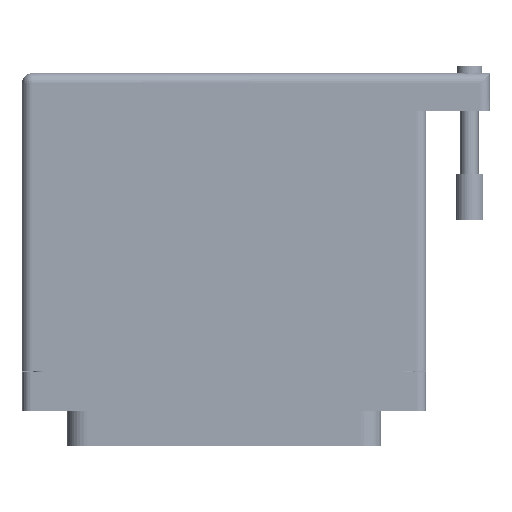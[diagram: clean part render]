
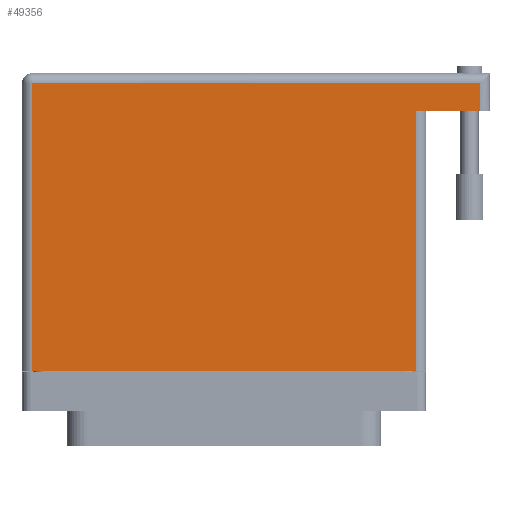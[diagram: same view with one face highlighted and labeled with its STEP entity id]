
A CAD part, front view. The second image highlights one B-rep face of the part: STEP entity #49356.
In plain terms, the highlighted face is planar.
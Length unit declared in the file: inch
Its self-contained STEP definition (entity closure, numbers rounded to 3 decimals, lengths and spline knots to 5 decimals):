
#3631 = CARTESIAN_POINT ( 'NONE',  ( 1.8125, 1.674, 0.765 ) ) ;
#5376 = DIRECTION ( 'NONE',  ( -1., 0., 0. ) ) ;
#6197 = ORIENTED_EDGE ( 'NONE', *, *, #26275, .F. ) ;
#10442 = CARTESIAN_POINT ( 'NONE',  ( -1.3775, -0.1, 0.765 ) ) ;
#16301 = CARTESIAN_POINT ( 'NONE',  ( -1.3775, 1.86, 0.765 ) ) ;
#18499 = CARTESIAN_POINT ( 'NONE',  ( -1.3775, 1.93, 0.765 ) ) ;
#18827 = VERTEX_POINT ( 'NONE', #66549 ) ;
#19673 = FACE_OUTER_BOUND ( 'NONE', #25398, .T. ) ;
#20328 = ORIENTED_EDGE ( 'NONE', *, *, #23964, .T. ) ;
#21923 = VECTOR ( 'NONE', #41911, 39.37008 ) ;
#23964 = EDGE_CURVE ( 'NONE', #54976, #90650, #58745, .T. ) ;
#24410 = VERTEX_POINT ( 'NONE', #43535 ) ;
#25398 = EDGE_LOOP ( 'NONE', ( #61426, #30986, #6197, #43374, #41675, #20328 ) ) ;
#26275 = EDGE_CURVE ( 'NONE', #24410, #18827, #43807, .T. ) ;
#28622 = CARTESIAN_POINT ( 'NONE',  ( -1.3075, 1.86, 0.765 ) ) ;
#28946 = CARTESIAN_POINT ( 'NONE',  ( 1.3075, -0.1, 0.765 ) ) ;
#30986 = ORIENTED_EDGE ( 'NONE', *, *, #32632, .T. ) ;
#32547 = VECTOR ( 'NONE', #81700, 39.37008 ) ;
#32632 = EDGE_CURVE ( 'NONE', #44425, #18827, #60925, .T. ) ;
#33595 = LINE ( 'NONE', #16301, #32547 ) ;
#36705 = EDGE_CURVE ( 'NONE', #46387, #54976, #33595, .T. ) ;
#38788 = LINE ( 'NONE', #10442, #55604 ) ;
#41675 = ORIENTED_EDGE ( 'NONE', *, *, #36705, .T. ) ;
#41911 = DIRECTION ( 'NONE',  ( 0., -1., 0. ) ) ;
#42209 = CARTESIAN_POINT ( 'NONE',  ( -1.3075, -0.1, 0.765 ) ) ;
#43374 = ORIENTED_EDGE ( 'NONE', *, *, #58482, .T. ) ;
#43535 = CARTESIAN_POINT ( 'NONE',  ( 1.7425, 1.674, 0.765 ) ) ;
#43807 = LINE ( 'NONE', #3631, #80760 ) ;
#44425 = VERTEX_POINT ( 'NONE', #28946 ) ;
#45221 = DIRECTION ( 'NONE',  ( -1., 0., 0. ) ) ;
#46387 = VERTEX_POINT ( 'NONE', #69286 ) ;
#47542 = DIRECTION ( 'NONE',  ( 0., 0., -1. ) ) ;
#49356 = ADVANCED_FACE ( 'NONE', ( #19673 ), #90427, .F. ) ;
#50839 = DIRECTION ( 'NONE',  ( 0., 1., 0. ) ) ;
#54976 = VERTEX_POINT ( 'NONE', #28622 ) ;
#55604 = VECTOR ( 'NONE', #74558, 39.37008 ) ;
#57719 = AXIS2_PLACEMENT_3D ( 'NONE', #18499, #47542, #5376 ) ;
#58482 = EDGE_CURVE ( 'NONE', #24410, #46387, #90675, .T. ) ;
#58745 = LINE ( 'NONE', #42209, #21923 ) ;
#60925 = LINE ( 'NONE', #63745, #77841 ) ;
#61426 = ORIENTED_EDGE ( 'NONE', *, *, #84565, .T. ) ;
#63745 = CARTESIAN_POINT ( 'NONE',  ( 1.3075, 1.674, 0.765 ) ) ;
#64791 = VECTOR ( 'NONE', #50839, 39.37008 ) ;
#66549 = CARTESIAN_POINT ( 'NONE',  ( 1.3075, 1.674, 0.765 ) ) ;
#69286 = CARTESIAN_POINT ( 'NONE',  ( 1.7425, 1.86, 0.765 ) ) ;
#71037 = DIRECTION ( 'NONE',  ( 0., 1., 0. ) ) ;
#74558 = DIRECTION ( 'NONE',  ( 1., 0., 0. ) ) ;
#77841 = VECTOR ( 'NONE', #71037, 39.37008 ) ;
#80760 = VECTOR ( 'NONE', #45221, 39.37008 ) ;
#81700 = DIRECTION ( 'NONE',  ( -1., 0., 0. ) ) ;
#84565 = EDGE_CURVE ( 'NONE', #90650, #44425, #38788, .T. ) ;
#86669 = CARTESIAN_POINT ( 'NONE',  ( -1.3075, -0.1, 0.765 ) ) ;
#87211 = CARTESIAN_POINT ( 'NONE',  ( 1.7425, 1.93, 0.765 ) ) ;
#90427 = PLANE ( 'NONE',  #57719 ) ;
#90650 = VERTEX_POINT ( 'NONE', #86669 ) ;
#90675 = LINE ( 'NONE', #87211, #64791 ) ;
